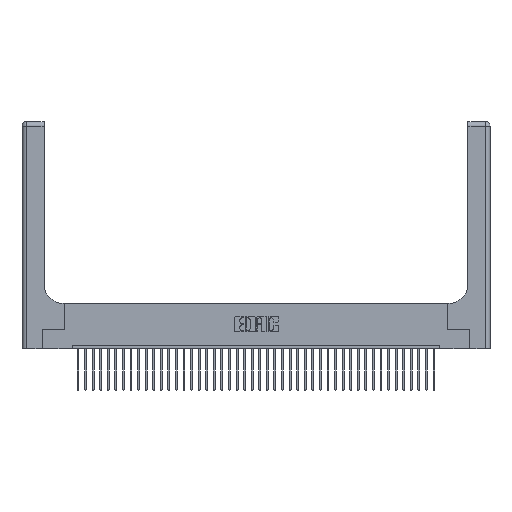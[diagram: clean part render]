
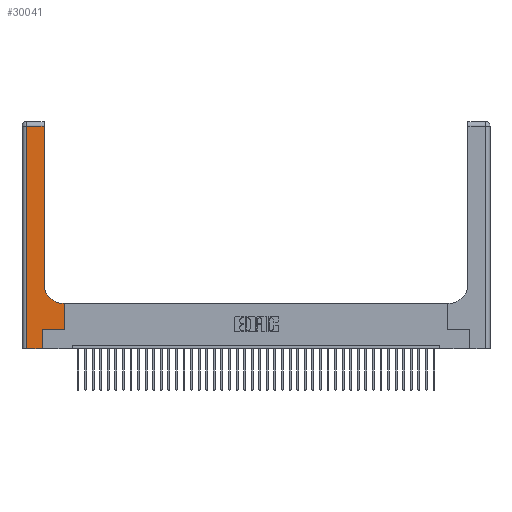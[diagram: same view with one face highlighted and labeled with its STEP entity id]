
A CAD part, top view. The second image highlights one B-rep face of the part: STEP entity #30041.
In plain terms, the highlighted planar face has unit normal (0, 0, 1).
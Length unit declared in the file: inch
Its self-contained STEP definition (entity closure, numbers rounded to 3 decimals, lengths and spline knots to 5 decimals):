
#183 = VERTEX_POINT ( 'NONE', #39396 ) ;
#197 = VERTEX_POINT ( 'NONE', #5055 ) ;
#340 = LINE ( 'NONE', #24055, #9615 ) ;
#415 = VERTEX_POINT ( 'NONE', #27754 ) ;
#533 = EDGE_CURVE ( 'NONE', #1996, #30244, #6730, .T. ) ;
#771 = CARTESIAN_POINT ( 'NONE',  ( 0.5585, 0.6, 0.37 ) ) ;
#1462 = CARTESIAN_POINT ( 'NONE',  ( 0.06, 2.94, 0.37 ) ) ;
#1996 = VERTEX_POINT ( 'NONE', #771 ) ;
#2008 = CARTESIAN_POINT ( 'NONE',  ( 0., 0., 0.37 ) ) ;
#2331 = ORIENTED_EDGE ( 'NONE', *, *, #39460, .T. ) ;
#3178 = CARTESIAN_POINT ( 'NONE',  ( 0.2915, 3., 0.37 ) ) ;
#3548 = PLANE ( 'NONE',  #34135 ) ;
#4070 = CIRCLE ( 'NONE', #40401, 0.25 ) ;
#4881 = VECTOR ( 'NONE', #38375, 39.37008 ) ;
#5055 = CARTESIAN_POINT ( 'NONE',  ( 0.06, 0., 0.37 ) ) ;
#5162 = LINE ( 'NONE', #3178, #24261 ) ;
#5846 = LINE ( 'NONE', #16493, #4881 ) ;
#6730 = LINE ( 'NONE', #28712, #39081 ) ;
#6854 = LINE ( 'NONE', #11978, #19590 ) ;
#7542 = VECTOR ( 'NONE', #39547, 39.37008 ) ;
#9155 = CARTESIAN_POINT ( 'NONE',  ( 0.5585, 0.25, 0.37 ) ) ;
#9391 = VERTEX_POINT ( 'NONE', #31431 ) ;
#9394 = EDGE_LOOP ( 'NONE', ( #29445, #20034, #18997, #24358, #24452, #2331, #38241, #12788, #21593 ) ) ;
#9453 = VERTEX_POINT ( 'NONE', #1462 ) ;
#9550 = CARTESIAN_POINT ( 'NONE',  ( 0., 3., 0.37 ) ) ;
#9615 = VECTOR ( 'NONE', #37550, 39.37008 ) ;
#10149 = EDGE_CURVE ( 'NONE', #197, #183, #16428, .T. ) ;
#10989 = CARTESIAN_POINT ( 'NONE',  ( 0.5415, 0.85, 0.37 ) ) ;
#11978 = CARTESIAN_POINT ( 'NONE',  ( 0.5585, 0.25, 0.37 ) ) ;
#12788 = ORIENTED_EDGE ( 'NONE', *, *, #533, .T. ) ;
#13815 = FACE_OUTER_BOUND ( 'NONE', #9394, .T. ) ;
#14891 = LINE ( 'NONE', #20801, #7542 ) ;
#16428 = LINE ( 'NONE', #2008, #40397 ) ;
#16493 = CARTESIAN_POINT ( 'NONE',  ( 0.06, 3., 0.37 ) ) ;
#17204 = CARTESIAN_POINT ( 'NONE',  ( 0.5415, 0.6, 0.37 ) ) ;
#17689 = LINE ( 'NONE', #18462, #26993 ) ;
#18462 = CARTESIAN_POINT ( 'NONE',  ( 0., 2.94, 0.37 ) ) ;
#18997 = ORIENTED_EDGE ( 'NONE', *, *, #37345, .T. ) ;
#19590 = VECTOR ( 'NONE', #40048, 39.37008 ) ;
#19707 = CARTESIAN_POINT ( 'NONE',  ( 0.269, 0.25, 0.37 ) ) ;
#19931 = EDGE_CURVE ( 'NONE', #415, #9391, #5162, .T. ) ;
#20034 = ORIENTED_EDGE ( 'NONE', *, *, #23493, .T. ) ;
#20801 = CARTESIAN_POINT ( 'NONE',  ( 0.269, 0.25, 0.37 ) ) ;
#21593 = ORIENTED_EDGE ( 'NONE', *, *, #30407, .T. ) ;
#23493 = EDGE_CURVE ( 'NONE', #9391, #9453, #17689, .T. ) ;
#24055 = CARTESIAN_POINT ( 'NONE',  ( 0.269, 0., 0.37 ) ) ;
#24261 = VECTOR ( 'NONE', #34390, 39.37008 ) ;
#24358 = ORIENTED_EDGE ( 'NONE', *, *, #10149, .T. ) ;
#24452 = ORIENTED_EDGE ( 'NONE', *, *, #38802, .T. ) ;
#25116 = DIRECTION ( 'NONE',  ( -1., 0., 0. ) ) ;
#26993 = VECTOR ( 'NONE', #40469, 39.37008 ) ;
#27754 = CARTESIAN_POINT ( 'NONE',  ( 0.2915, 0.85, 0.37 ) ) ;
#28712 = CARTESIAN_POINT ( 'NONE',  ( 0.2915, 0.6, 0.37 ) ) ;
#29445 = ORIENTED_EDGE ( 'NONE', *, *, #19931, .T. ) ;
#29973 = VERTEX_POINT ( 'NONE', #9155 ) ;
#30041 = ADVANCED_FACE ( 'NONE', ( #13815 ), #3548, .F. ) ;
#30244 = VERTEX_POINT ( 'NONE', #17204 ) ;
#30407 = EDGE_CURVE ( 'NONE', #30244, #415, #4070, .T. ) ;
#31362 = DIRECTION ( 'NONE',  ( -1., 0., 0. ) ) ;
#31431 = CARTESIAN_POINT ( 'NONE',  ( 0.2915, 2.94, 0.37 ) ) ;
#31921 = DIRECTION ( 'NONE',  ( 0., 0., -1. ) ) ;
#32739 = VERTEX_POINT ( 'NONE', #19707 ) ;
#32914 = DIRECTION ( 'NONE',  ( 1., 0., 0. ) ) ;
#34135 = AXIS2_PLACEMENT_3D ( 'NONE', #9550, #31921, #31362 ) ;
#34390 = DIRECTION ( 'NONE',  ( 0., 1., 0. ) ) ;
#35770 = DIRECTION ( 'NONE',  ( 0., 0., -1. ) ) ;
#36198 = DIRECTION ( 'NONE',  ( 1., 0., 0. ) ) ;
#37034 = EDGE_CURVE ( 'NONE', #29973, #1996, #6854, .T. ) ;
#37345 = EDGE_CURVE ( 'NONE', #9453, #197, #5846, .T. ) ;
#37550 = DIRECTION ( 'NONE',  ( 0., 1., 0. ) ) ;
#38241 = ORIENTED_EDGE ( 'NONE', *, *, #37034, .T. ) ;
#38375 = DIRECTION ( 'NONE',  ( 0., -1., 0. ) ) ;
#38802 = EDGE_CURVE ( 'NONE', #183, #32739, #340, .T. ) ;
#39081 = VECTOR ( 'NONE', #25116, 39.37008 ) ;
#39396 = CARTESIAN_POINT ( 'NONE',  ( 0.269, 0., 0.37 ) ) ;
#39460 = EDGE_CURVE ( 'NONE', #32739, #29973, #14891, .T. ) ;
#39547 = DIRECTION ( 'NONE',  ( 1., 0., 0. ) ) ;
#40048 = DIRECTION ( 'NONE',  ( 0., 1., 0. ) ) ;
#40397 = VECTOR ( 'NONE', #36198, 39.37008 ) ;
#40401 = AXIS2_PLACEMENT_3D ( 'NONE', #10989, #35770, #32914 ) ;
#40469 = DIRECTION ( 'NONE',  ( -1., 0., 0. ) ) ;
